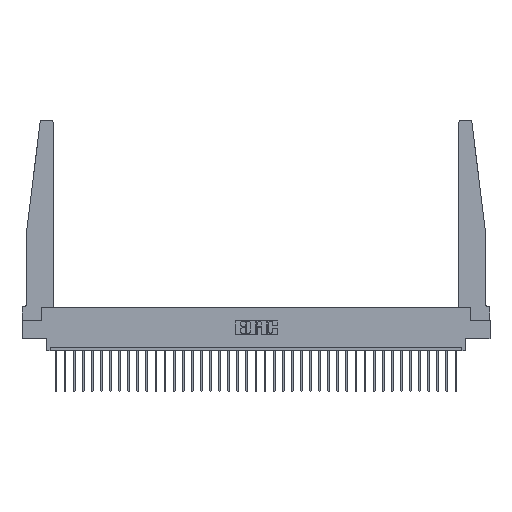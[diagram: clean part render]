
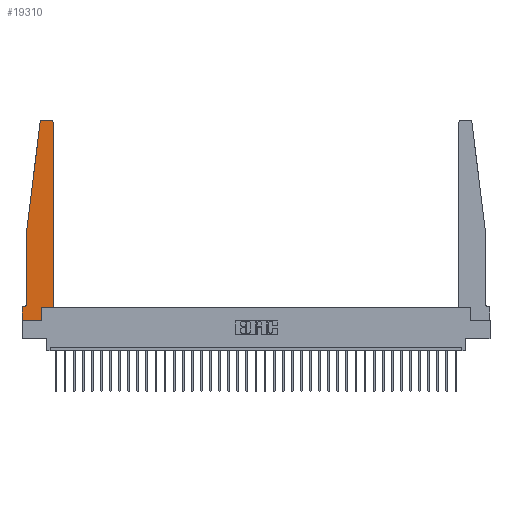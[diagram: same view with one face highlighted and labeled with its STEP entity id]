
A CAD part, top view. The second image highlights one B-rep face of the part: STEP entity #19310.
In plain terms, the highlighted planar face has unit normal (0, 0, 1).
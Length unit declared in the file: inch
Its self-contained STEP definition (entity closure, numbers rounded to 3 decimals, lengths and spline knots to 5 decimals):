
#9 = CARTESIAN_POINT ( 'NONE',  ( 0.425, 0.18, 0.37 ) ) ;
#644 = LINE ( 'NONE', #27492, #13154 ) ;
#900 = CARTESIAN_POINT ( 'NONE',  ( 0.27653, 2.72, 0.37 ) ) ;
#1167 = LINE ( 'NONE', #3022, #22774 ) ;
#2427 = CARTESIAN_POINT ( 'NONE',  ( 0., 0., 0.37 ) ) ;
#3022 = CARTESIAN_POINT ( 'NONE',  ( 0.425, 0.18, 0.37 ) ) ;
#3526 = DIRECTION ( 'NONE',  ( -1., 0., 0. ) ) ;
#4686 = DIRECTION ( 'NONE',  ( 1., 0., 0. ) ) ;
#4914 = DIRECTION ( 'NONE',  ( 0., -1., 0. ) ) ;
#6098 = ORIENTED_EDGE ( 'NONE', *, *, #28372, .T. ) ;
#6754 = CARTESIAN_POINT ( 'NONE',  ( 0., 0., 0.37 ) ) ;
#6806 = VECTOR ( 'NONE', #4914, 39.37008 ) ;
#6899 = LINE ( 'NONE', #28755, #23803 ) ;
#6937 = LINE ( 'NONE', #23736, #26605 ) ;
#7725 = LINE ( 'NONE', #10345, #12035 ) ;
#8074 = EDGE_CURVE ( 'NONE', #27889, #8381, #6937, .T. ) ;
#8381 = VERTEX_POINT ( 'NONE', #9505 ) ;
#9505 = CARTESIAN_POINT ( 'NONE',  ( 0.27653, 2.75, 0.37 ) ) ;
#9592 = DIRECTION ( 'NONE',  ( 0., 0., 1. ) ) ;
#10171 = EDGE_LOOP ( 'NONE', ( #13420, #13344, #6098, #15760, #19995, #27818, #30691, #11643, #27268, #13800, #10921, #27488 ) ) ;
#10345 = CARTESIAN_POINT ( 'NONE',  ( 0.065, 1.25, 0.37 ) ) ;
#10921 = ORIENTED_EDGE ( 'NONE', *, *, #23041, .T. ) ;
#10930 = LINE ( 'NONE', #26998, #24739 ) ;
#11043 = CARTESIAN_POINT ( 'NONE',  ( 0.395, 2.75, 0.37 ) ) ;
#11325 = DIRECTION ( 'NONE',  ( 0., 1., 0. ) ) ;
#11643 = ORIENTED_EDGE ( 'NONE', *, *, #28056, .T. ) ;
#11991 = CIRCLE ( 'NONE', #19050, 0.03 ) ;
#12035 = VECTOR ( 'NONE', #20144, 39.37008 ) ;
#12056 = DIRECTION ( 'NONE',  ( 0., 0., 1. ) ) ;
#12472 = CIRCLE ( 'NONE', #24733, 0.03 ) ;
#12967 = DIRECTION ( 'NONE',  ( 1., 0., 0. ) ) ;
#13154 = VECTOR ( 'NONE', #29890, 39.37008 ) ;
#13252 = DIRECTION ( 'NONE',  ( 0., 0., -1. ) ) ;
#13258 = DIRECTION ( 'NONE',  ( 1., 0., 0. ) ) ;
#13344 = ORIENTED_EDGE ( 'NONE', *, *, #27686, .T. ) ;
#13420 = ORIENTED_EDGE ( 'NONE', *, *, #8074, .T. ) ;
#13786 = EDGE_CURVE ( 'NONE', #31930, #15511, #16197, .T. ) ;
#13800 = ORIENTED_EDGE ( 'NONE', *, *, #16282, .T. ) ;
#14676 = CARTESIAN_POINT ( 'NONE',  ( 0., 0.1875, 0.37 ) ) ;
#15511 = VERTEX_POINT ( 'NONE', #28326 ) ;
#15596 = CARTESIAN_POINT ( 'NONE',  ( 0.2605, 0., 0.37 ) ) ;
#15760 = ORIENTED_EDGE ( 'NONE', *, *, #19229, .T. ) ;
#15943 = LINE ( 'NONE', #6754, #25831 ) ;
#16197 = LINE ( 'NONE', #2427, #6806 ) ;
#16214 = VERTEX_POINT ( 'NONE', #16877 ) ;
#16261 = CARTESIAN_POINT ( 'NONE',  ( 0., 0.1875, 0.37 ) ) ;
#16282 = EDGE_CURVE ( 'NONE', #31211, #23173, #1167, .T. ) ;
#16528 = VERTEX_POINT ( 'NONE', #15596 ) ;
#16877 = CARTESIAN_POINT ( 'NONE',  ( 0.015, 0.1875, 0.37 ) ) ;
#17225 = DIRECTION ( 'NONE',  ( 1., 0., 0. ) ) ;
#18062 = VERTEX_POINT ( 'NONE', #19377 ) ;
#18135 = CARTESIAN_POINT ( 'NONE',  ( 0.425, 0.18, 0.37 ) ) ;
#18413 = DIRECTION ( 'NONE',  ( 0., 0., 1. ) ) ;
#18990 = VECTOR ( 'NONE', #32298, 39.37008 ) ;
#19050 = AXIS2_PLACEMENT_3D ( 'NONE', #32304, #9592, #4686 ) ;
#19229 = EDGE_CURVE ( 'NONE', #32192, #19562, #10930, .T. ) ;
#19310 = ADVANCED_FACE ( 'NONE', ( #21997 ), #29829, .T. ) ;
#19377 = CARTESIAN_POINT ( 'NONE',  ( 0.24675, 2.72367, 0.37 ) ) ;
#19379 = CARTESIAN_POINT ( 'NONE',  ( 0.2605, 0.18, 0.37 ) ) ;
#19562 = VERTEX_POINT ( 'NONE', #30821 ) ;
#19995 = ORIENTED_EDGE ( 'NONE', *, *, #30616, .T. ) ;
#20144 = DIRECTION ( 'NONE',  ( -0.122, -0.992, 0. ) ) ;
#21092 = EDGE_CURVE ( 'NONE', #25041, #27889, #11991, .T. ) ;
#21280 = EDGE_CURVE ( 'NONE', #16214, #31930, #644, .T. ) ;
#21541 = EDGE_CURVE ( 'NONE', #16528, #31211, #6899, .T. ) ;
#21752 = CARTESIAN_POINT ( 'NONE',  ( 0.425, 2.72, 0.37 ) ) ;
#21997 = FACE_OUTER_BOUND ( 'NONE', #10171, .T. ) ;
#22774 = VECTOR ( 'NONE', #12967, 39.37008 ) ;
#23041 = EDGE_CURVE ( 'NONE', #23173, #25041, #23739, .T. ) ;
#23173 = VERTEX_POINT ( 'NONE', #18135 ) ;
#23736 = CARTESIAN_POINT ( 'NONE',  ( 0.25, 2.75, 0.37 ) ) ;
#23739 = LINE ( 'NONE', #9, #18990 ) ;
#23803 = VECTOR ( 'NONE', #11325, 39.37008 ) ;
#24621 = DIRECTION ( 'NONE',  ( 0., -1., 0. ) ) ;
#24733 = AXIS2_PLACEMENT_3D ( 'NONE', #900, #18413, #13258 ) ;
#24739 = VECTOR ( 'NONE', #24621, 39.37008 ) ;
#25041 = VERTEX_POINT ( 'NONE', #21752 ) ;
#25308 = CIRCLE ( 'NONE', #25991, 0.05 ) ;
#25831 = VECTOR ( 'NONE', #26534, 39.37008 ) ;
#25991 = AXIS2_PLACEMENT_3D ( 'NONE', #28269, #13252, #30762 ) ;
#26534 = DIRECTION ( 'NONE',  ( 1., 0., 0. ) ) ;
#26605 = VECTOR ( 'NONE', #3526, 39.37008 ) ;
#26998 = CARTESIAN_POINT ( 'NONE',  ( 0.065, 1.25, 0.37 ) ) ;
#27038 = AXIS2_PLACEMENT_3D ( 'NONE', #14676, #12056, #17225 ) ;
#27268 = ORIENTED_EDGE ( 'NONE', *, *, #21541, .T. ) ;
#27488 = ORIENTED_EDGE ( 'NONE', *, *, #21092, .T. ) ;
#27492 = CARTESIAN_POINT ( 'NONE',  ( 0.065, 0.1875, 0.37 ) ) ;
#27686 = EDGE_CURVE ( 'NONE', #8381, #18062, #12472, .T. ) ;
#27818 = ORIENTED_EDGE ( 'NONE', *, *, #21280, .T. ) ;
#27889 = VERTEX_POINT ( 'NONE', #11043 ) ;
#28056 = EDGE_CURVE ( 'NONE', #15511, #16528, #15943, .T. ) ;
#28269 = CARTESIAN_POINT ( 'NONE',  ( 0.015, 0.2375, 0.37 ) ) ;
#28326 = CARTESIAN_POINT ( 'NONE',  ( 0., 0., 0.37 ) ) ;
#28372 = EDGE_CURVE ( 'NONE', #18062, #32192, #7725, .T. ) ;
#28755 = CARTESIAN_POINT ( 'NONE',  ( 0.2605, 0.18, 0.37 ) ) ;
#29829 = PLANE ( 'NONE',  #27038 ) ;
#29890 = DIRECTION ( 'NONE',  ( -1., 0., 0. ) ) ;
#30616 = EDGE_CURVE ( 'NONE', #19562, #16214, #25308, .T. ) ;
#30691 = ORIENTED_EDGE ( 'NONE', *, *, #13786, .T. ) ;
#30762 = DIRECTION ( 'NONE',  ( -1., 0., 0. ) ) ;
#30821 = CARTESIAN_POINT ( 'NONE',  ( 0.065, 0.2375, 0.37 ) ) ;
#31211 = VERTEX_POINT ( 'NONE', #19379 ) ;
#31930 = VERTEX_POINT ( 'NONE', #16261 ) ;
#32192 = VERTEX_POINT ( 'NONE', #32431 ) ;
#32298 = DIRECTION ( 'NONE',  ( 0., 1., 0. ) ) ;
#32304 = CARTESIAN_POINT ( 'NONE',  ( 0.395, 2.72, 0.37 ) ) ;
#32431 = CARTESIAN_POINT ( 'NONE',  ( 0.065, 1.25, 0.37 ) ) ;
